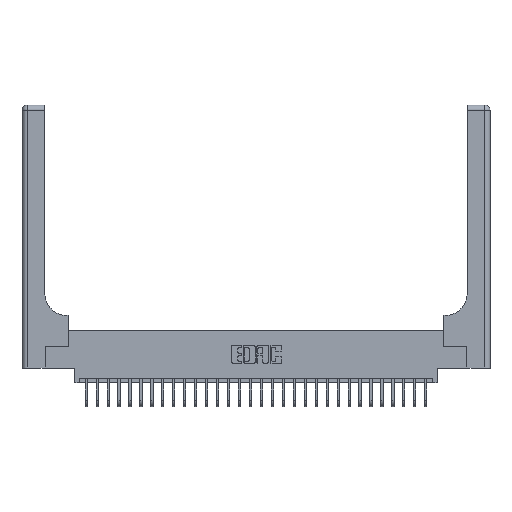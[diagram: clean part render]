
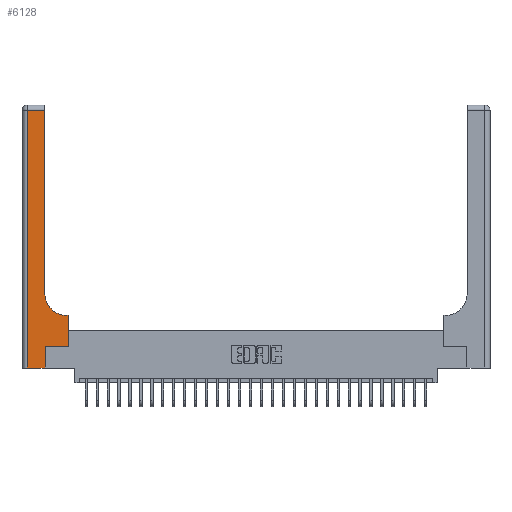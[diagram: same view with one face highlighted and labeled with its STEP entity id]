
A CAD part, top view. The second image highlights one B-rep face of the part: STEP entity #6128.
In plain terms, the highlighted planar face has unit normal (0, 0, 1).
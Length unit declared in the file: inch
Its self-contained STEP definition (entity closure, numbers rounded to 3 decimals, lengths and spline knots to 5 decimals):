
#912 = CARTESIAN_POINT ( 'NONE',  ( 0.265, 0., 0.37 ) ) ;
#961 = VERTEX_POINT ( 'NONE', #8932 ) ;
#1378 = VERTEX_POINT ( 'NONE', #14575 ) ;
#1388 = DIRECTION ( 'NONE',  ( 0., 0., -1. ) ) ;
#1413 = EDGE_CURVE ( 'NONE', #14676, #2950, #22453, .T. ) ;
#2537 = DIRECTION ( 'NONE',  ( 0., -1., 0. ) ) ;
#2950 = VERTEX_POINT ( 'NONE', #18908 ) ;
#3010 = CARTESIAN_POINT ( 'NONE',  ( 0., 0., 0.37 ) ) ;
#3201 = VERTEX_POINT ( 'NONE', #3259 ) ;
#3259 = CARTESIAN_POINT ( 'NONE',  ( 0.528, 0.6, 0.37 ) ) ;
#3314 = CARTESIAN_POINT ( 'NONE',  ( 0.528, 0.25, 0.37 ) ) ;
#3689 = VECTOR ( 'NONE', #24263, 39.37008 ) ;
#3986 = CARTESIAN_POINT ( 'NONE',  ( 0.265, 0.25, 0.37 ) ) ;
#4088 = DIRECTION ( 'NONE',  ( 1., 0., 0. ) ) ;
#4305 = VECTOR ( 'NONE', #2537, 39.37008 ) ;
#4381 = CARTESIAN_POINT ( 'NONE',  ( 0.26, 0.6, 0.37 ) ) ;
#4429 = CARTESIAN_POINT ( 'NONE',  ( 0.26, 0.85, 0.37 ) ) ;
#4447 = LINE ( 'NONE', #3010, #20791 ) ;
#4528 = VECTOR ( 'NONE', #11457, 39.37008 ) ;
#4862 = VECTOR ( 'NONE', #27372, 39.37008 ) ;
#5027 = DIRECTION ( 'NONE',  ( 0., 0., -1. ) ) ;
#5447 = VECTOR ( 'NONE', #12651, 39.37008 ) ;
#5771 = CARTESIAN_POINT ( 'NONE',  ( 0.51, 0.85, 0.37 ) ) ;
#5962 = AXIS2_PLACEMENT_3D ( 'NONE', #5771, #1388, #28352 ) ;
#6075 = ORIENTED_EDGE ( 'NONE', *, *, #7367, .T. ) ;
#6106 = FACE_OUTER_BOUND ( 'NONE', #8444, .T. ) ;
#6128 = ADVANCED_FACE ( 'NONE', ( #6106 ), #11809, .F. ) ;
#7367 = EDGE_CURVE ( 'NONE', #15867, #3201, #26755, .T. ) ;
#8026 = ORIENTED_EDGE ( 'NONE', *, *, #1413, .T. ) ;
#8306 = CARTESIAN_POINT ( 'NONE',  ( 0., 2.94, 0.37 ) ) ;
#8444 = EDGE_LOOP ( 'NONE', ( #8026, #28716, #22321, #22563, #24989, #16737, #6075, #26436, #20170 ) ) ;
#8932 = CARTESIAN_POINT ( 'NONE',  ( 0.06, 2.94, 0.37 ) ) ;
#10483 = EDGE_CURVE ( 'NONE', #25537, #13326, #4447, .T. ) ;
#10898 = EDGE_CURVE ( 'NONE', #13326, #1378, #25122, .T. ) ;
#10939 = CIRCLE ( 'NONE', #5962, 0.25 ) ;
#11457 = DIRECTION ( 'NONE',  ( -1., 0., 0. ) ) ;
#11809 = PLANE ( 'NONE',  #16930 ) ;
#12651 = DIRECTION ( 'NONE',  ( 0., 1., 0. ) ) ;
#12652 = EDGE_CURVE ( 'NONE', #3201, #22456, #14439, .T. ) ;
#13326 = VERTEX_POINT ( 'NONE', #912 ) ;
#14016 = CARTESIAN_POINT ( 'NONE',  ( 0.265, 0., 0.37 ) ) ;
#14439 = LINE ( 'NONE', #4381, #4528 ) ;
#14465 = VECTOR ( 'NONE', #4088, 39.37008 ) ;
#14575 = CARTESIAN_POINT ( 'NONE',  ( 0.265, 0.25, 0.37 ) ) ;
#14676 = VERTEX_POINT ( 'NONE', #4429 ) ;
#15867 = VERTEX_POINT ( 'NONE', #18833 ) ;
#16118 = CARTESIAN_POINT ( 'NONE',  ( 0.06, 3., 0.37 ) ) ;
#16308 = CARTESIAN_POINT ( 'NONE',  ( 0., 3., 0.37 ) ) ;
#16737 = ORIENTED_EDGE ( 'NONE', *, *, #18116, .T. ) ;
#16930 = AXIS2_PLACEMENT_3D ( 'NONE', #16308, #5027, #23180 ) ;
#18116 = EDGE_CURVE ( 'NONE', #1378, #15867, #19836, .T. ) ;
#18149 = LINE ( 'NONE', #16118, #4305 ) ;
#18833 = CARTESIAN_POINT ( 'NONE',  ( 0.528, 0.25, 0.37 ) ) ;
#18908 = CARTESIAN_POINT ( 'NONE',  ( 0.26, 2.94, 0.37 ) ) ;
#19836 = LINE ( 'NONE', #3986, #14465 ) ;
#20170 = ORIENTED_EDGE ( 'NONE', *, *, #28372, .T. ) ;
#20206 = CARTESIAN_POINT ( 'NONE',  ( 0.51, 0.6, 0.37 ) ) ;
#20791 = VECTOR ( 'NONE', #25632, 39.37008 ) ;
#21468 = LINE ( 'NONE', #8306, #3689 ) ;
#21578 = DIRECTION ( 'NONE',  ( 0., 1., 0. ) ) ;
#21949 = EDGE_CURVE ( 'NONE', #961, #25537, #18149, .T. ) ;
#22321 = ORIENTED_EDGE ( 'NONE', *, *, #21949, .T. ) ;
#22453 = LINE ( 'NONE', #28347, #5447 ) ;
#22456 = VERTEX_POINT ( 'NONE', #20206 ) ;
#22563 = ORIENTED_EDGE ( 'NONE', *, *, #10483, .T. ) ;
#23180 = DIRECTION ( 'NONE',  ( -1., 0., 0. ) ) ;
#24263 = DIRECTION ( 'NONE',  ( -1., 0., 0. ) ) ;
#24989 = ORIENTED_EDGE ( 'NONE', *, *, #10898, .T. ) ;
#25003 = VECTOR ( 'NONE', #21578, 39.37008 ) ;
#25122 = LINE ( 'NONE', #14016, #4862 ) ;
#25499 = EDGE_CURVE ( 'NONE', #2950, #961, #21468, .T. ) ;
#25537 = VERTEX_POINT ( 'NONE', #26445 ) ;
#25632 = DIRECTION ( 'NONE',  ( 1., 0., 0. ) ) ;
#26436 = ORIENTED_EDGE ( 'NONE', *, *, #12652, .T. ) ;
#26445 = CARTESIAN_POINT ( 'NONE',  ( 0.06, 0., 0.37 ) ) ;
#26755 = LINE ( 'NONE', #3314, #25003 ) ;
#27372 = DIRECTION ( 'NONE',  ( 0., 1., 0. ) ) ;
#28347 = CARTESIAN_POINT ( 'NONE',  ( 0.26, 3., 0.37 ) ) ;
#28352 = DIRECTION ( 'NONE',  ( 1., 0., 0. ) ) ;
#28372 = EDGE_CURVE ( 'NONE', #22456, #14676, #10939, .T. ) ;
#28716 = ORIENTED_EDGE ( 'NONE', *, *, #25499, .T. ) ;
